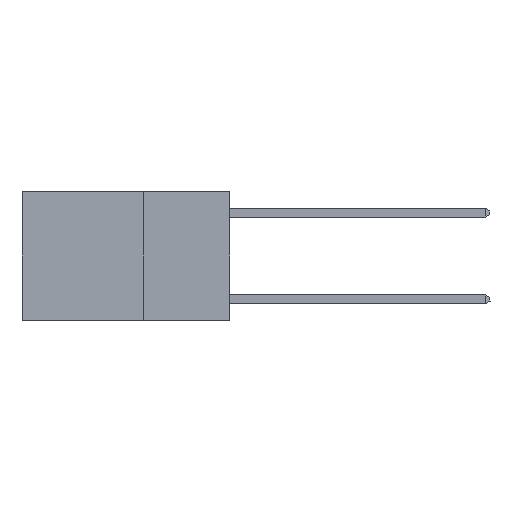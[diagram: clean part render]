
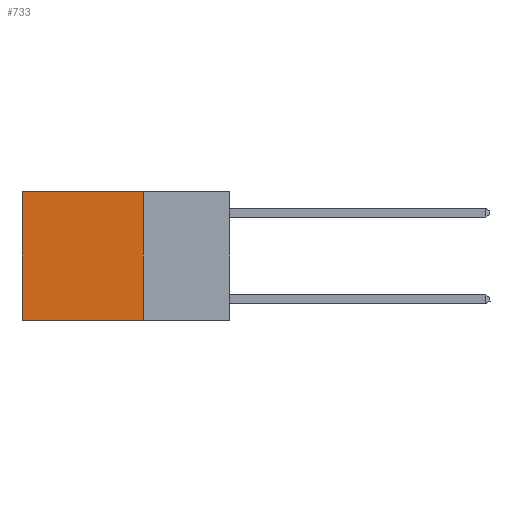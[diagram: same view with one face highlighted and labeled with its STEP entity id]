
A CAD part, left-side view. The second image highlights one B-rep face of the part: STEP entity #733.
In plain terms, the highlighted planar face has unit normal (-1, 0, 0).
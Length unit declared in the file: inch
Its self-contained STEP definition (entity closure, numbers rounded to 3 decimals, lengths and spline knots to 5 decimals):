
#129 = EDGE_CURVE ( 'NONE', #12190, #7260, #9691, .T. ) ;
#569 = VECTOR ( 'NONE', #10270, 39.37008 ) ;
#733 = ADVANCED_FACE ( 'NONE', ( #11812 ), #3057, .F. ) ;
#940 = CARTESIAN_POINT ( 'NONE',  ( 0.2625, 0.25, 0. ) ) ;
#1821 = DIRECTION ( 'NONE',  ( 1., 0., 0. ) ) ;
#2398 = CARTESIAN_POINT ( 'NONE',  ( 0.2625, 0.25, -0.37 ) ) ;
#2600 = EDGE_CURVE ( 'NONE', #15370, #6157, #5832, .T. ) ;
#3017 = DIRECTION ( 'NONE',  ( 0., 0., -1. ) ) ;
#3057 = PLANE ( 'NONE',  #7744 ) ;
#4513 = VECTOR ( 'NONE', #12538, 39.37008 ) ;
#4558 = ORIENTED_EDGE ( 'NONE', *, *, #129, .T. ) ;
#4823 = EDGE_CURVE ( 'NONE', #6157, #7260, #5147, .T. ) ;
#4859 = ORIENTED_EDGE ( 'NONE', *, *, #4823, .F. ) ;
#5147 = LINE ( 'NONE', #6957, #4513 ) ;
#5638 = VECTOR ( 'NONE', #3017, 39.37008 ) ;
#5832 = LINE ( 'NONE', #940, #6263 ) ;
#6157 = VERTEX_POINT ( 'NONE', #2398 ) ;
#6263 = VECTOR ( 'NONE', #10248, 39.37008 ) ;
#6913 = LINE ( 'NONE', #7728, #569 ) ;
#6957 = CARTESIAN_POINT ( 'NONE',  ( 0.2625, 0.25, -0.37 ) ) ;
#7260 = VERTEX_POINT ( 'NONE', #13531 ) ;
#7728 = CARTESIAN_POINT ( 'NONE',  ( 0.2625, 0.25, 0. ) ) ;
#7744 = AXIS2_PLACEMENT_3D ( 'NONE', #11450, #1821, #16883 ) ;
#8219 = ORIENTED_EDGE ( 'NONE', *, *, #2600, .F. ) ;
#9122 = ORIENTED_EDGE ( 'NONE', *, *, #12576, .T. ) ;
#9691 = LINE ( 'NONE', #13977, #5638 ) ;
#10248 = DIRECTION ( 'NONE',  ( 0., 0., -1. ) ) ;
#10270 = DIRECTION ( 'NONE',  ( 0., 1., 0. ) ) ;
#11450 = CARTESIAN_POINT ( 'NONE',  ( 0.2625, 0.25, 0. ) ) ;
#11590 = CARTESIAN_POINT ( 'NONE',  ( 0.2625, 0.6, 0. ) ) ;
#11812 = FACE_OUTER_BOUND ( 'NONE', #16412, .T. ) ;
#12190 = VERTEX_POINT ( 'NONE', #11590 ) ;
#12538 = DIRECTION ( 'NONE',  ( 0., 1., 0. ) ) ;
#12576 = EDGE_CURVE ( 'NONE', #15370, #12190, #6913, .T. ) ;
#13377 = CARTESIAN_POINT ( 'NONE',  ( 0.2625, 0.25, 0. ) ) ;
#13531 = CARTESIAN_POINT ( 'NONE',  ( 0.2625, 0.6, -0.37 ) ) ;
#13977 = CARTESIAN_POINT ( 'NONE',  ( 0.2625, 0.6, 0. ) ) ;
#15370 = VERTEX_POINT ( 'NONE', #13377 ) ;
#16412 = EDGE_LOOP ( 'NONE', ( #4558, #4859, #8219, #9122 ) ) ;
#16883 = DIRECTION ( 'NONE',  ( 0., 0., -1. ) ) ;
